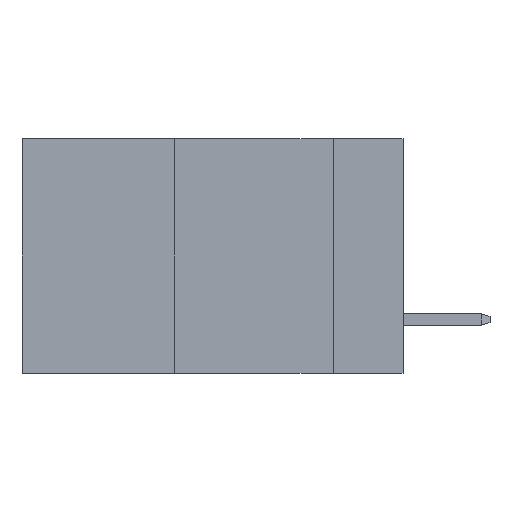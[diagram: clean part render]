
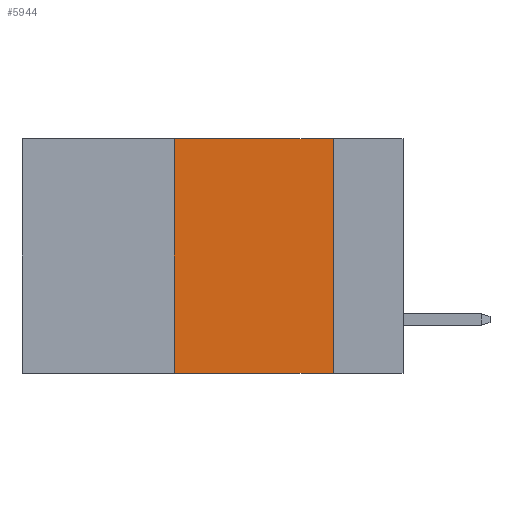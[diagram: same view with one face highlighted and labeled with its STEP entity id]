
A CAD part, left-side view. The second image highlights one B-rep face of the part: STEP entity #5944.
In plain terms, the highlighted planar face has unit normal (-1, 0, 0).
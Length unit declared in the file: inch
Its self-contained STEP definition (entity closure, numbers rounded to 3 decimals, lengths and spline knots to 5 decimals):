
#194 = DIRECTION ( 'NONE',  ( 0., 0., 1. ) ) ;
#208 = EDGE_CURVE ( 'NONE', #9180, #3255, #6641, .T. ) ;
#606 = DIRECTION ( 'NONE',  ( 0., 0., -1. ) ) ;
#783 = CARTESIAN_POINT ( 'NONE',  ( 0., 0.6, -0.37 ) ) ;
#1069 = LINE ( 'NONE', #7564, #7674 ) ;
#1078 = VERTEX_POINT ( 'NONE', #8163 ) ;
#1335 = DIRECTION ( 'NONE',  ( 1., 0., 0. ) ) ;
#1925 = ORIENTED_EDGE ( 'NONE', *, *, #8747, .F. ) ;
#2043 = ORIENTED_EDGE ( 'NONE', *, *, #6619, .F. ) ;
#2137 = CARTESIAN_POINT ( 'NONE',  ( 0., 0.11, 0. ) ) ;
#2451 = EDGE_LOOP ( 'NONE', ( #1925, #5725, #2043, #8794 ) ) ;
#3107 = EDGE_CURVE ( 'NONE', #1078, #8439, #5667, .T. ) ;
#3145 = CARTESIAN_POINT ( 'NONE',  ( 0., 0.11, -0.37 ) ) ;
#3255 = VERTEX_POINT ( 'NONE', #3145 ) ;
#3393 = LINE ( 'NONE', #2137, #7343 ) ;
#3841 = CARTESIAN_POINT ( 'NONE',  ( 0., 0.11, 0. ) ) ;
#4940 = CARTESIAN_POINT ( 'NONE',  ( 0., 0.6, 0. ) ) ;
#5005 = FACE_OUTER_BOUND ( 'NONE', #2451, .T. ) ;
#5242 = DIRECTION ( 'NONE',  ( 0., -1., 0. ) ) ;
#5667 = LINE ( 'NONE', #4940, #8417 ) ;
#5725 = ORIENTED_EDGE ( 'NONE', *, *, #3107, .F. ) ;
#5944 = ADVANCED_FACE ( 'NONE', ( #5005 ), #6506, .F. ) ;
#6506 = PLANE ( 'NONE',  #8321 ) ;
#6536 = DIRECTION ( 'NONE',  ( 0., 0., -1. ) ) ;
#6619 = EDGE_CURVE ( 'NONE', #9180, #1078, #1069, .T. ) ;
#6641 = LINE ( 'NONE', #783, #9098 ) ;
#7343 = VECTOR ( 'NONE', #6536, 39.37008 ) ;
#7564 = CARTESIAN_POINT ( 'NONE',  ( 0., 0.36, 0. ) ) ;
#7674 = VECTOR ( 'NONE', #194, 39.37008 ) ;
#7896 = DIRECTION ( 'NONE',  ( 0., -1., 0. ) ) ;
#7966 = CARTESIAN_POINT ( 'NONE',  ( 0., 0.6, 0. ) ) ;
#8163 = CARTESIAN_POINT ( 'NONE',  ( 0., 0.36, 0. ) ) ;
#8321 = AXIS2_PLACEMENT_3D ( 'NONE', #7966, #1335, #606 ) ;
#8417 = VECTOR ( 'NONE', #7896, 39.37008 ) ;
#8439 = VERTEX_POINT ( 'NONE', #3841 ) ;
#8747 = EDGE_CURVE ( 'NONE', #8439, #3255, #3393, .T. ) ;
#8794 = ORIENTED_EDGE ( 'NONE', *, *, #208, .T. ) ;
#9098 = VECTOR ( 'NONE', #5242, 39.37008 ) ;
#9180 = VERTEX_POINT ( 'NONE', #9348 ) ;
#9348 = CARTESIAN_POINT ( 'NONE',  ( 0., 0.36, -0.37 ) ) ;
